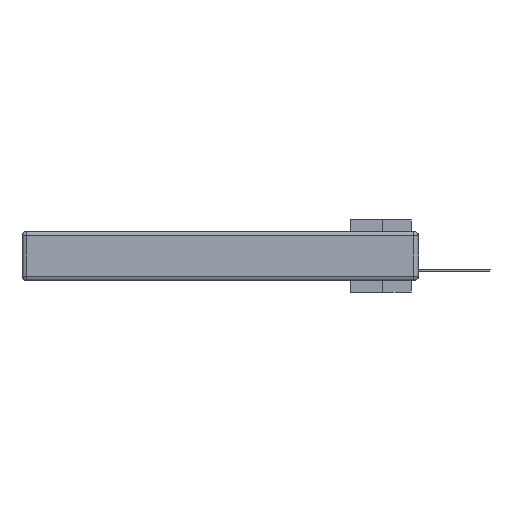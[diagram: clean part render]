
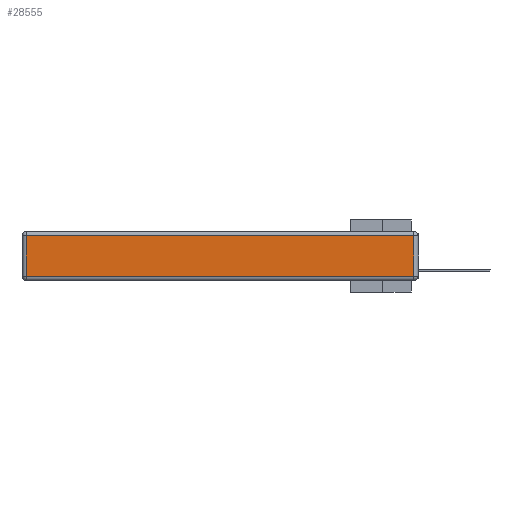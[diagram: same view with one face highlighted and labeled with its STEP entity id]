
A CAD part, left-side view. The second image highlights one B-rep face of the part: STEP entity #28555.
In plain terms, the highlighted planar face has unit normal (-1, 0, 0).
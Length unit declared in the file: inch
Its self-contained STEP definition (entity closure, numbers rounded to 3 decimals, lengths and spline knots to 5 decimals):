
#668 = CARTESIAN_POINT ( 'NONE',  ( 0., 0., -0.343 ) ) ;
#1718 = EDGE_CURVE ( 'NONE', #4168, #25276, #9932, .T. ) ;
#1880 = EDGE_LOOP ( 'NONE', ( #21830, #12691, #4484, #19318 ) ) ;
#2153 = CARTESIAN_POINT ( 'NONE',  ( 0., 0.03, -0.313 ) ) ;
#4168 = VERTEX_POINT ( 'NONE', #2153 ) ;
#4484 = ORIENTED_EDGE ( 'NONE', *, *, #24891, .T. ) ;
#4961 = DIRECTION ( 'NONE',  ( -1., 0., 0. ) ) ;
#6329 = LINE ( 'NONE', #6606, #19960 ) ;
#6606 = CARTESIAN_POINT ( 'NONE',  ( 0., 2.75, -0.03 ) ) ;
#7167 = PLANE ( 'NONE',  #8825 ) ;
#8825 = AXIS2_PLACEMENT_3D ( 'NONE', #668, #4961, #20610 ) ;
#9932 = LINE ( 'NONE', #16551, #24968 ) ;
#12435 = CARTESIAN_POINT ( 'NONE',  ( 0., 2.72, -0.03 ) ) ;
#12691 = ORIENTED_EDGE ( 'NONE', *, *, #1718, .T. ) ;
#12911 = DIRECTION ( 'NONE',  ( 0., -1., 0. ) ) ;
#14600 = DIRECTION ( 'NONE',  ( 0., 0., -1. ) ) ;
#15052 = VERTEX_POINT ( 'NONE', #18877 ) ;
#16418 = VERTEX_POINT ( 'NONE', #12435 ) ;
#16551 = CARTESIAN_POINT ( 'NONE',  ( 0., 0.03, -0.343 ) ) ;
#16955 = LINE ( 'NONE', #23752, #22237 ) ;
#17215 = CARTESIAN_POINT ( 'NONE',  ( 0., 0.03, -0.03 ) ) ;
#17276 = EDGE_CURVE ( 'NONE', #15052, #4168, #19675, .T. ) ;
#18268 = FACE_OUTER_BOUND ( 'NONE', #1880, .T. ) ;
#18877 = CARTESIAN_POINT ( 'NONE',  ( 0., 2.72, -0.313 ) ) ;
#19318 = ORIENTED_EDGE ( 'NONE', *, *, #22027, .T. ) ;
#19675 = LINE ( 'NONE', #28255, #28569 ) ;
#19960 = VECTOR ( 'NONE', #24189, 39.37008 ) ;
#20610 = DIRECTION ( 'NONE',  ( 0., 0., 1. ) ) ;
#21830 = ORIENTED_EDGE ( 'NONE', *, *, #17276, .T. ) ;
#22027 = EDGE_CURVE ( 'NONE', #16418, #15052, #16955, .T. ) ;
#22237 = VECTOR ( 'NONE', #14600, 39.37008 ) ;
#22917 = DIRECTION ( 'NONE',  ( 0., 0., 1. ) ) ;
#23752 = CARTESIAN_POINT ( 'NONE',  ( 0., 2.72, -0.343 ) ) ;
#24189 = DIRECTION ( 'NONE',  ( 0., 1., 0. ) ) ;
#24891 = EDGE_CURVE ( 'NONE', #25276, #16418, #6329, .T. ) ;
#24968 = VECTOR ( 'NONE', #22917, 39.37008 ) ;
#25276 = VERTEX_POINT ( 'NONE', #17215 ) ;
#28255 = CARTESIAN_POINT ( 'NONE',  ( 0., 0., -0.313 ) ) ;
#28555 = ADVANCED_FACE ( 'NONE', ( #18268 ), #7167, .T. ) ;
#28569 = VECTOR ( 'NONE', #12911, 39.37008 ) ;
